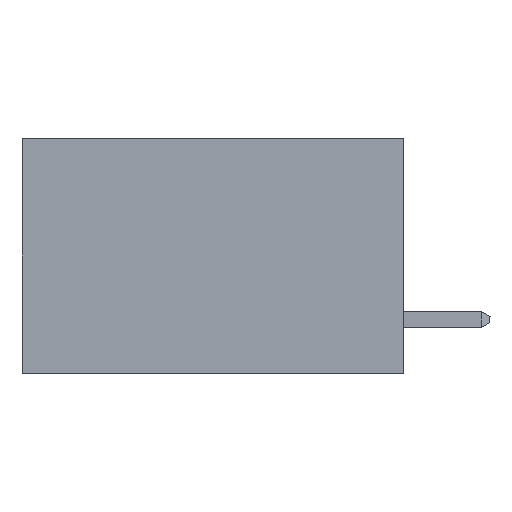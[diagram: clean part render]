
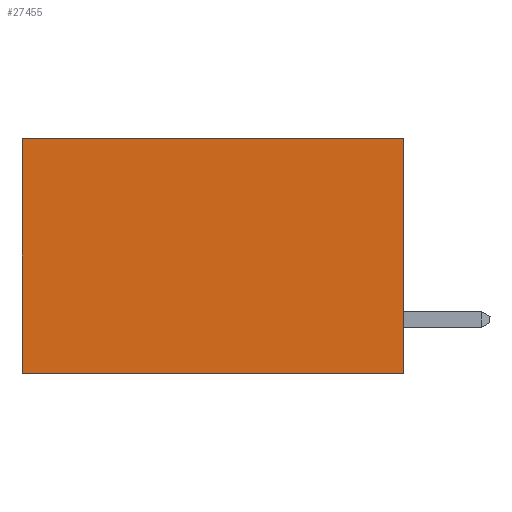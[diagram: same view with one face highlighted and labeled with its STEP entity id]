
A CAD part, left-side view. The second image highlights one B-rep face of the part: STEP entity #27455.
In plain terms, the highlighted planar face has unit normal (-1, 0, 0).
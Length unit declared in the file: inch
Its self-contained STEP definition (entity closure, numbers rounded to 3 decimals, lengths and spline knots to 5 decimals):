
#1910 = DIRECTION ( 'NONE',  ( 0., 1., 0. ) ) ;
#3285 = ORIENTED_EDGE ( 'NONE', *, *, #27829, .F. ) ;
#3691 = CARTESIAN_POINT ( 'NONE',  ( 0.2875, 0., 0. ) ) ;
#4611 = CARTESIAN_POINT ( 'NONE',  ( 0.2875, 0.6, -0.37 ) ) ;
#5461 = DIRECTION ( 'NONE',  ( 0., 0., -1. ) ) ;
#6040 = VECTOR ( 'NONE', #5461, 39.37008 ) ;
#7279 = EDGE_CURVE ( 'NONE', #17701, #18395, #30472, .T. ) ;
#7586 = CARTESIAN_POINT ( 'NONE',  ( 0.2875, 0., 0. ) ) ;
#9210 = CARTESIAN_POINT ( 'NONE',  ( 0.2875, 0., 0. ) ) ;
#9705 = AXIS2_PLACEMENT_3D ( 'NONE', #3691, #23447, #30499 ) ;
#10162 = VECTOR ( 'NONE', #1910, 39.37008 ) ;
#10983 = CARTESIAN_POINT ( 'NONE',  ( 0.2875, 0., -0.37 ) ) ;
#11907 = LINE ( 'NONE', #10983, #16094 ) ;
#13548 = DIRECTION ( 'NONE',  ( 0., 1., 0. ) ) ;
#14969 = CARTESIAN_POINT ( 'NONE',  ( 0.2875, 0.6, 0. ) ) ;
#16094 = VECTOR ( 'NONE', #13548, 39.37008 ) ;
#17418 = CARTESIAN_POINT ( 'NONE',  ( 0.2875, 0., -0.37 ) ) ;
#17530 = CARTESIAN_POINT ( 'NONE',  ( 0.2875, 0.6, 0. ) ) ;
#17701 = VERTEX_POINT ( 'NONE', #14969 ) ;
#18194 = PLANE ( 'NONE',  #9705 ) ;
#18395 = VERTEX_POINT ( 'NONE', #4611 ) ;
#18738 = VECTOR ( 'NONE', #19970, 39.37008 ) ;
#18948 = FACE_OUTER_BOUND ( 'NONE', #29083, .T. ) ;
#19970 = DIRECTION ( 'NONE',  ( 0., 0., -1. ) ) ;
#20170 = VERTEX_POINT ( 'NONE', #7586 ) ;
#20219 = ORIENTED_EDGE ( 'NONE', *, *, #27611, .T. ) ;
#22321 = EDGE_CURVE ( 'NONE', #30488, #18395, #11907, .T. ) ;
#22554 = CARTESIAN_POINT ( 'NONE',  ( 0.2875, 0., 0. ) ) ;
#23447 = DIRECTION ( 'NONE',  ( 1., 0., 0. ) ) ;
#23828 = ORIENTED_EDGE ( 'NONE', *, *, #22321, .F. ) ;
#25371 = LINE ( 'NONE', #22554, #6040 ) ;
#27455 = ADVANCED_FACE ( 'NONE', ( #18948 ), #18194, .F. ) ;
#27611 = EDGE_CURVE ( 'NONE', #20170, #17701, #30268, .T. ) ;
#27829 = EDGE_CURVE ( 'NONE', #20170, #30488, #25371, .T. ) ;
#29083 = EDGE_LOOP ( 'NONE', ( #29707, #23828, #3285, #20219 ) ) ;
#29707 = ORIENTED_EDGE ( 'NONE', *, *, #7279, .T. ) ;
#30268 = LINE ( 'NONE', #9210, #10162 ) ;
#30472 = LINE ( 'NONE', #17530, #18738 ) ;
#30488 = VERTEX_POINT ( 'NONE', #17418 ) ;
#30499 = DIRECTION ( 'NONE',  ( 0., 0., -1. ) ) ;
